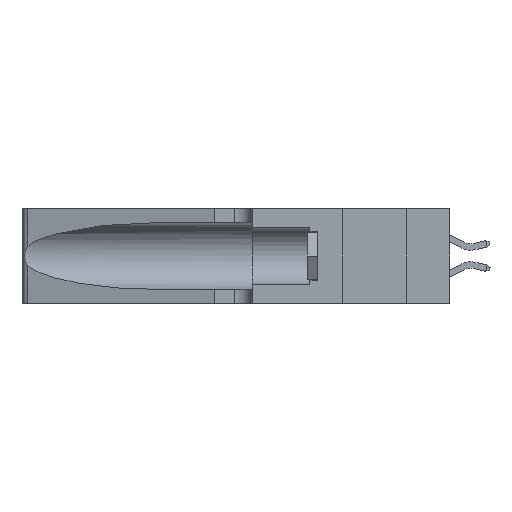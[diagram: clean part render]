
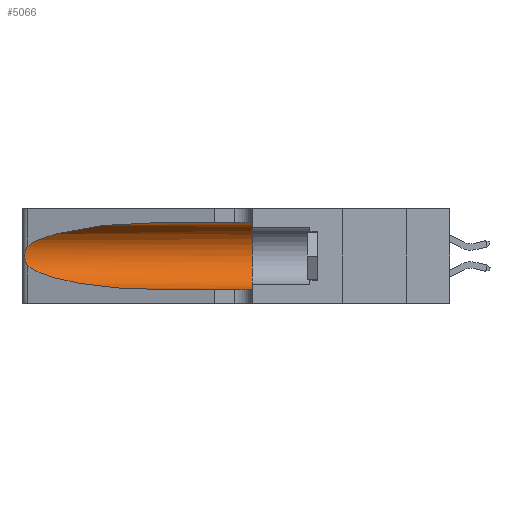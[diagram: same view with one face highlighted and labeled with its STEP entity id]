
A CAD part, left-side view. The second image highlights one B-rep face of the part: STEP entity #5066.
In plain terms, the highlighted cylindrical face has radius 3.308 mm (diameter 6.617 mm), a partial arc.
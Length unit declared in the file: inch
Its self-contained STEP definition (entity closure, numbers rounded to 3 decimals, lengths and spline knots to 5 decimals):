
#241 =( BOUNDED_CURVE ( )  B_SPLINE_CURVE ( 3, ( #13581, #749, #24580, #7569 ),
 .UNSPECIFIED., .F., .T. ) 
 B_SPLINE_CURVE_WITH_KNOTS ( ( 4, 4 ),
 ( 1.5708, 2.84003 ),
 .UNSPECIFIED. ) 
 CURVE ( )  GEOMETRIC_REPRESENTATION_ITEM ( )  RATIONAL_B_SPLINE_CURVE ( ( 1., 0.87, 0.87, 1. ) ) 
 REPRESENTATION_ITEM ( '' )  );
#551 = CARTESIAN_POINT ( 'NONE',  ( 0.26018, 1.23835, 0.19895 ) ) ;
#747 = CARTESIAN_POINT ( 'NONE',  ( 0.25789, 1.23486, 0.15765 ) ) ;
#749 = CARTESIAN_POINT ( 'NONE',  ( 0.18966, 0.96281, 0.31525 ) ) ;
#1802 = CARTESIAN_POINT ( 'NONE',  ( 0.25487, 1.22718, 0.22369 ) ) ;
#2222 = VERTEX_POINT ( 'NONE', #21101 ) ;
#2564 = CYLINDRICAL_SURFACE ( 'NONE', #16553, 0.13025 ) ;
#2796 = CARTESIAN_POINT ( 'NONE',  ( 0.26075, 1.23896, 0.19203 ) ) ;
#2860 = CARTESIAN_POINT ( 'NONE',  ( 0.2373, 1.15595, 0.08982 ) ) ;
#2991 = CARTESIAN_POINT ( 'NONE',  ( 0.25555, 1.22993, 0.14849 ) ) ;
#4340 = VERTEX_POINT ( 'NONE', #25788 ) ;
#4465 = DIRECTION ( 'NONE',  ( 0., -1., 0. ) ) ;
#5066 = ADVANCED_FACE ( 'NONE', ( #25374 ), #2564, .F. ) ;
#5214 = B_SPLINE_CURVE_WITH_KNOTS ( 'NONE', 3,
 ( #1802, #25207, #19325, #8536, #15097, #551, #2796, #22013, #17879, #26380, #747, #21740, #2991, #18055 ),
 .UNSPECIFIED., .F., .F.,
 ( 4, 2, 2, 2, 2, 2, 4 ),
 ( 0., 0.00027, 0.00053, 0.00107, 0.0016, 0.00187, 0.00214 ),
 .UNSPECIFIED. ) ;
#5263 = CARTESIAN_POINT ( 'NONE',  ( 0.1305, 1.61858, 0.185 ) ) ;
#7283 = VECTOR ( 'NONE', #4465, 39.37008 ) ;
#7569 = CARTESIAN_POINT ( 'NONE',  ( 0.25487, 1.22718, 0.22369 ) ) ;
#8424 = ORIENTED_EDGE ( 'NONE', *, *, #11007, .F. ) ;
#8536 = CARTESIAN_POINT ( 'NONE',  ( 0.25787, 1.23484, 0.2124 ) ) ;
#8598 = CARTESIAN_POINT ( 'NONE',  ( 0.1305, 0.35, 0.185 ) ) ;
#8681 = LINE ( 'NONE', #16716, #17393 ) ;
#9023 = VERTEX_POINT ( 'NONE', #13184 ) ;
#9763 = ORIENTED_EDGE ( 'NONE', *, *, #10847, .T. ) ;
#9989 = ORIENTED_EDGE ( 'NONE', *, *, #19879, .T. ) ;
#10838 = DIRECTION ( 'NONE',  ( 0., 1., 0. ) ) ;
#10847 = EDGE_CURVE ( 'NONE', #9023, #16788, #5214, .T. ) ;
#11007 = EDGE_CURVE ( 'NONE', #2222, #4340, #20060, .T. ) ;
#12070 = AXIS2_PLACEMENT_3D ( 'NONE', #8598, #10838, #19393 ) ;
#12078 = ORIENTED_EDGE ( 'NONE', *, *, #23745, .F. ) ;
#12146 = CARTESIAN_POINT ( 'NONE',  ( 0.1305, 0.72297, 0.05475 ) ) ;
#12327 = CARTESIAN_POINT ( 'NONE',  ( 0.18966, 0.96281, 0.05475 ) ) ;
#13184 = CARTESIAN_POINT ( 'NONE',  ( 0.25487, 1.22718, 0.22369 ) ) ;
#13479 = CIRCLE ( 'NONE', #12070, 0.13025 ) ;
#13581 = CARTESIAN_POINT ( 'NONE',  ( 0.1305, 0.72297, 0.31525 ) ) ;
#14176 = DIRECTION ( 'NONE',  ( 0., -1., 0. ) ) ;
#14999 = EDGE_LOOP ( 'NONE', ( #9989, #9763, #19476, #23269, #12078, #8424 ) ) ;
#15097 = CARTESIAN_POINT ( 'NONE',  ( 0.25854, 1.2359, 0.20912 ) ) ;
#15351 = CARTESIAN_POINT ( 'NONE',  ( 0.25487, 1.22718, 0.14631 ) ) ;
#15369 = EDGE_CURVE ( 'NONE', #16788, #17411, #21562, .T. ) ;
#16553 = AXIS2_PLACEMENT_3D ( 'NONE', #5263, #14176, #22417 ) ;
#16716 = CARTESIAN_POINT ( 'NONE',  ( 0.1305, 1.61858, 0.05475 ) ) ;
#16788 = VERTEX_POINT ( 'NONE', #15351 ) ;
#17393 = VECTOR ( 'NONE', #27287, 39.37008 ) ;
#17411 = VERTEX_POINT ( 'NONE', #27173 ) ;
#17879 = CARTESIAN_POINT ( 'NONE',  ( 0.26017, 1.23833, 0.17102 ) ) ;
#18055 = CARTESIAN_POINT ( 'NONE',  ( 0.25487, 1.22718, 0.14631 ) ) ;
#19325 = CARTESIAN_POINT ( 'NONE',  ( 0.25639, 1.23184, 0.21858 ) ) ;
#19393 = DIRECTION ( 'NONE',  ( 0., 0., 1. ) ) ;
#19476 = ORIENTED_EDGE ( 'NONE', *, *, #15369, .T. ) ;
#19879 = EDGE_CURVE ( 'NONE', #2222, #9023, #241, .T. ) ;
#20060 = LINE ( 'NONE', #21537, #7283 ) ;
#20920 = VERTEX_POINT ( 'NONE', #26031 ) ;
#21101 = CARTESIAN_POINT ( 'NONE',  ( 0.1305, 0.72297, 0.31525 ) ) ;
#21537 = CARTESIAN_POINT ( 'NONE',  ( 0.1305, 1.61858, 0.31525 ) ) ;
#21562 =( BOUNDED_CURVE ( )  B_SPLINE_CURVE ( 3, ( #21881, #2860, #12327, #12146 ),
 .UNSPECIFIED., .F., .F. ) 
 B_SPLINE_CURVE_WITH_KNOTS ( ( 4, 4 ),
 ( 3.44316, 4.71239 ),
 .UNSPECIFIED. ) 
 CURVE ( )  GEOMETRIC_REPRESENTATION_ITEM ( )  RATIONAL_B_SPLINE_CURVE ( ( 1., 0.87, 0.87, 1. ) ) 
 REPRESENTATION_ITEM ( '' )  );
#21740 = CARTESIAN_POINT ( 'NONE',  ( 0.25639, 1.23186, 0.15144 ) ) ;
#21881 = CARTESIAN_POINT ( 'NONE',  ( 0.25487, 1.22718, 0.14631 ) ) ;
#22013 = CARTESIAN_POINT ( 'NONE',  ( 0.26075, 1.23896, 0.178 ) ) ;
#22417 = DIRECTION ( 'NONE',  ( 0., 0., -1. ) ) ;
#23269 = ORIENTED_EDGE ( 'NONE', *, *, #25693, .T. ) ;
#23745 = EDGE_CURVE ( 'NONE', #4340, #20920, #13479, .T. ) ;
#24580 = CARTESIAN_POINT ( 'NONE',  ( 0.2373, 1.15595, 0.28018 ) ) ;
#25207 = CARTESIAN_POINT ( 'NONE',  ( 0.25555, 1.22994, 0.2215 ) ) ;
#25374 = FACE_OUTER_BOUND ( 'NONE', #14999, .T. ) ;
#25693 = EDGE_CURVE ( 'NONE', #17411, #20920, #8681, .T. ) ;
#25788 = CARTESIAN_POINT ( 'NONE',  ( 0.1305, 0.35, 0.31525 ) ) ;
#26031 = CARTESIAN_POINT ( 'NONE',  ( 0.1305, 0.35, 0.05475 ) ) ;
#26380 = CARTESIAN_POINT ( 'NONE',  ( 0.25856, 1.23593, 0.16098 ) ) ;
#27173 = CARTESIAN_POINT ( 'NONE',  ( 0.1305, 0.72297, 0.05475 ) ) ;
#27287 = DIRECTION ( 'NONE',  ( 0., -1., 0. ) ) ;
